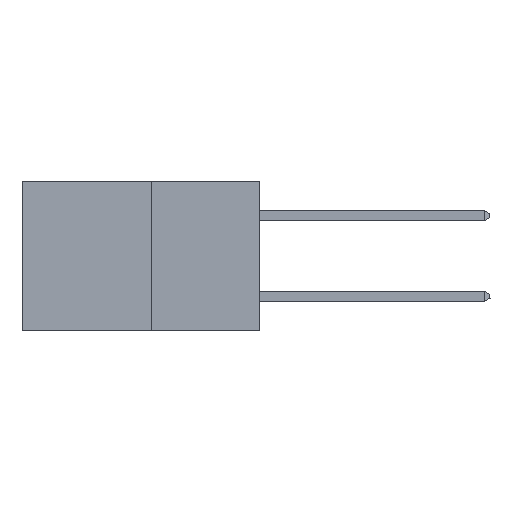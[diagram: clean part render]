
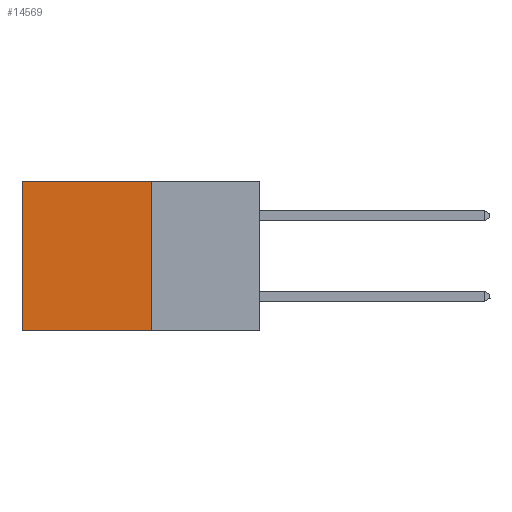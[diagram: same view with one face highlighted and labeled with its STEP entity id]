
A CAD part, left-side view. The second image highlights one B-rep face of the part: STEP entity #14569.
In plain terms, the highlighted planar face has unit normal (-1, 0, 0).
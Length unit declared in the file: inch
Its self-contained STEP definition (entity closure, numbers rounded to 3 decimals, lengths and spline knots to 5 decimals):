
#2986 = CARTESIAN_POINT ( 'NONE',  ( 0.277, 0.27, -0.37 ) ) ;
#3816 = EDGE_CURVE ( 'NONE', #18152, #20562, #12002, .T. ) ;
#4378 = CARTESIAN_POINT ( 'NONE',  ( 0.277, 0.27, -0.37 ) ) ;
#5732 = VERTEX_POINT ( 'NONE', #20014 ) ;
#6345 = DIRECTION ( 'NONE',  ( 0., 0., -1. ) ) ;
#6516 = CARTESIAN_POINT ( 'NONE',  ( 0.277, 0.27, -0.37 ) ) ;
#7448 = CARTESIAN_POINT ( 'NONE',  ( 0.277, 0.27, -0.37 ) ) ;
#9854 = ORIENTED_EDGE ( 'NONE', *, *, #16120, .F. ) ;
#10846 = LINE ( 'NONE', #11131, #21879 ) ;
#11131 = CARTESIAN_POINT ( 'NONE',  ( 0.277, 0.27, 0. ) ) ;
#11368 = VECTOR ( 'NONE', #16316, 39.37008 ) ;
#12002 = LINE ( 'NONE', #15216, #11368 ) ;
#12710 = VECTOR ( 'NONE', #24583, 39.37008 ) ;
#13600 = VECTOR ( 'NONE', #17331, 39.37008 ) ;
#14569 = ADVANCED_FACE ( 'NONE', ( #20158 ), #23915, .F. ) ;
#14887 = EDGE_CURVE ( 'NONE', #5732, #18152, #10846, .T. ) ;
#15216 = CARTESIAN_POINT ( 'NONE',  ( 0.277, 0.59, -0.37 ) ) ;
#15498 = EDGE_CURVE ( 'NONE', #5732, #20514, #23102, .T. ) ;
#16120 = EDGE_CURVE ( 'NONE', #20514, #20562, #24638, .T. ) ;
#16316 = DIRECTION ( 'NONE',  ( 0., 0., -1. ) ) ;
#16809 = ORIENTED_EDGE ( 'NONE', *, *, #15498, .F. ) ;
#17080 = ORIENTED_EDGE ( 'NONE', *, *, #3816, .T. ) ;
#17331 = DIRECTION ( 'NONE',  ( 0., 1., 0. ) ) ;
#17428 = CARTESIAN_POINT ( 'NONE',  ( 0.277, 0.59, 0. ) ) ;
#18114 = DIRECTION ( 'NONE',  ( 1., 0., 0. ) ) ;
#18152 = VERTEX_POINT ( 'NONE', #17428 ) ;
#18330 = EDGE_LOOP ( 'NONE', ( #17080, #9854, #16809, #24872 ) ) ;
#18447 = CARTESIAN_POINT ( 'NONE',  ( 0.277, 0.59, -0.37 ) ) ;
#20014 = CARTESIAN_POINT ( 'NONE',  ( 0.277, 0.27, 0. ) ) ;
#20158 = FACE_OUTER_BOUND ( 'NONE', #18330, .T. ) ;
#20514 = VERTEX_POINT ( 'NONE', #6516 ) ;
#20562 = VERTEX_POINT ( 'NONE', #18447 ) ;
#21879 = VECTOR ( 'NONE', #22871, 39.37008 ) ;
#22871 = DIRECTION ( 'NONE',  ( 0., 1., 0. ) ) ;
#23102 = LINE ( 'NONE', #2986, #12710 ) ;
#23851 = AXIS2_PLACEMENT_3D ( 'NONE', #4378, #18114, #6345 ) ;
#23915 = PLANE ( 'NONE',  #23851 ) ;
#24583 = DIRECTION ( 'NONE',  ( 0., 0., -1. ) ) ;
#24638 = LINE ( 'NONE', #7448, #13600 ) ;
#24872 = ORIENTED_EDGE ( 'NONE', *, *, #14887, .T. ) ;
